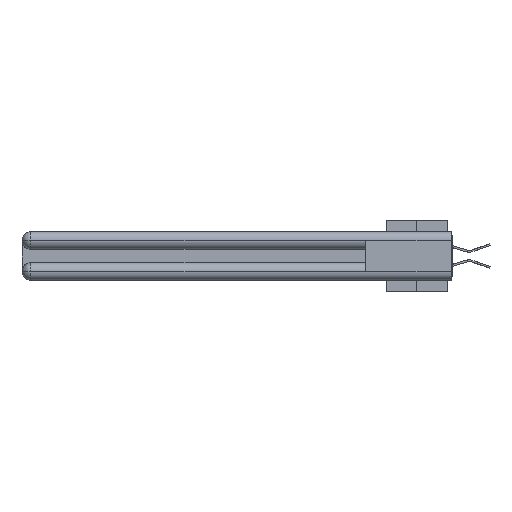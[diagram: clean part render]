
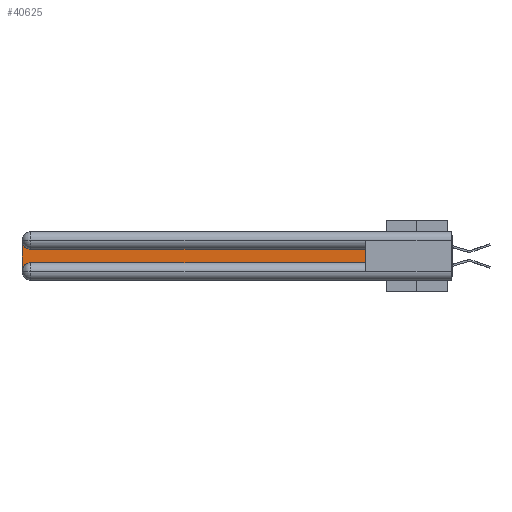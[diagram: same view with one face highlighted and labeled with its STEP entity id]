
A CAD part, left-side view. The second image highlights one B-rep face of the part: STEP entity #40625.
In plain terms, the highlighted planar face has unit normal (-1, 0, 0).
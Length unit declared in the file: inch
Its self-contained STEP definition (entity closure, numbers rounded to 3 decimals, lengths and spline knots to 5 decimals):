
#57 = VERTEX_POINT ( 'NONE', #10335 ) ;
#139 = CIRCLE ( 'NONE', #19681, 0.06 ) ;
#1927 = CARTESIAN_POINT ( 'NONE',  ( 0.075, 3., -0.0625 ) ) ;
#2142 = LINE ( 'NONE', #23280, #25725 ) ;
#4754 = CARTESIAN_POINT ( 'NONE',  ( 0.075, 2.94, -0.1225 ) ) ;
#4976 = EDGE_CURVE ( 'NONE', #7288, #57, #2142, .T. ) ;
#4984 = DIRECTION ( 'NONE',  ( 1., 0., 0. ) ) ;
#5056 = VERTEX_POINT ( 'NONE', #16002 ) ;
#5619 = DIRECTION ( 'NONE',  ( 1., 0., 0. ) ) ;
#6218 = DIRECTION ( 'NONE',  ( 0., 1., 0. ) ) ;
#6311 = CARTESIAN_POINT ( 'NONE',  ( 0.075, 3., -0.1225 ) ) ;
#6501 = FACE_OUTER_BOUND ( 'NONE', #9477, .T. ) ;
#6801 = PLANE ( 'NONE',  #38234 ) ;
#7288 = VERTEX_POINT ( 'NONE', #23890 ) ;
#8958 = CARTESIAN_POINT ( 'NONE',  ( 0.075, 2.94, -0.2175 ) ) ;
#9477 = EDGE_LOOP ( 'NONE', ( #12114, #29584, #33956, #25727, #12480, #31195 ) ) ;
#9574 = EDGE_CURVE ( 'NONE', #57, #26640, #20072, .T. ) ;
#10335 = CARTESIAN_POINT ( 'NONE',  ( 0.075, 0.6, -0.1225 ) ) ;
#10534 = VECTOR ( 'NONE', #45537, 39.37008 ) ;
#12114 = ORIENTED_EDGE ( 'NONE', *, *, #9574, .T. ) ;
#12480 = ORIENTED_EDGE ( 'NONE', *, *, #40442, .T. ) ;
#13454 = CARTESIAN_POINT ( 'NONE',  ( 0.075, 0.6, -0.1225 ) ) ;
#15430 = CARTESIAN_POINT ( 'NONE',  ( 0.075, 2.94, -0.2775 ) ) ;
#15576 = DIRECTION ( 'NONE',  ( 0., 0., -1. ) ) ;
#16002 = CARTESIAN_POINT ( 'NONE',  ( 0.075, 3., -0.2775 ) ) ;
#16155 = DIRECTION ( 'NONE',  ( 0., 0., 1. ) ) ;
#18025 = LINE ( 'NONE', #19202, #10534 ) ;
#19202 = CARTESIAN_POINT ( 'NONE',  ( 0.075, 0.6, -0.2175 ) ) ;
#19458 = EDGE_CURVE ( 'NONE', #36359, #5056, #25043, .T. ) ;
#19681 = AXIS2_PLACEMENT_3D ( 'NONE', #39004, #5619, #27857 ) ;
#20072 = LINE ( 'NONE', #13454, #34528 ) ;
#22904 = EDGE_CURVE ( 'NONE', #5056, #37103, #37385, .T. ) ;
#23280 = CARTESIAN_POINT ( 'NONE',  ( 0.075, 0.6, -0.2175 ) ) ;
#23890 = CARTESIAN_POINT ( 'NONE',  ( 0.075, 0.6, -0.2175 ) ) ;
#25043 = LINE ( 'NONE', #37708, #26204 ) ;
#25725 = VECTOR ( 'NONE', #16155, 39.37008 ) ;
#25727 = ORIENTED_EDGE ( 'NONE', *, *, #22904, .T. ) ;
#26204 = VECTOR ( 'NONE', #15576, 39.37008 ) ;
#26640 = VERTEX_POINT ( 'NONE', #4754 ) ;
#27463 = AXIS2_PLACEMENT_3D ( 'NONE', #15430, #4984, #30773 ) ;
#27857 = DIRECTION ( 'NONE',  ( 0., 0., -1. ) ) ;
#29584 = ORIENTED_EDGE ( 'NONE', *, *, #41077, .T. ) ;
#30773 = DIRECTION ( 'NONE',  ( 0., 0., -1. ) ) ;
#31195 = ORIENTED_EDGE ( 'NONE', *, *, #4976, .T. ) ;
#33956 = ORIENTED_EDGE ( 'NONE', *, *, #19458, .T. ) ;
#34528 = VECTOR ( 'NONE', #6218, 39.37008 ) ;
#36322 = DIRECTION ( 'NONE',  ( 1., 0., 0. ) ) ;
#36359 = VERTEX_POINT ( 'NONE', #1927 ) ;
#37103 = VERTEX_POINT ( 'NONE', #8958 ) ;
#37385 = CIRCLE ( 'NONE', #27463, 0.06 ) ;
#37708 = CARTESIAN_POINT ( 'NONE',  ( 0.075, 3., -0.2175 ) ) ;
#38234 = AXIS2_PLACEMENT_3D ( 'NONE', #6311, #36322, #39220 ) ;
#39004 = CARTESIAN_POINT ( 'NONE',  ( 0.075, 2.94, -0.0625 ) ) ;
#39220 = DIRECTION ( 'NONE',  ( 0., 0., -1. ) ) ;
#40442 = EDGE_CURVE ( 'NONE', #37103, #7288, #18025, .T. ) ;
#40625 = ADVANCED_FACE ( 'NONE', ( #6501 ), #6801, .F. ) ;
#41077 = EDGE_CURVE ( 'NONE', #26640, #36359, #139, .T. ) ;
#45537 = DIRECTION ( 'NONE',  ( 0., -1., 0. ) ) ;
